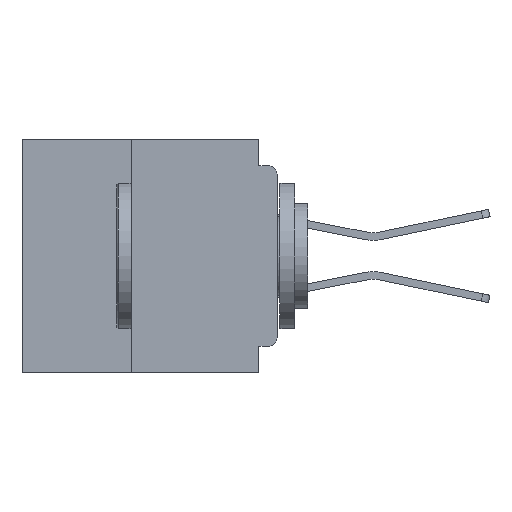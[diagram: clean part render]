
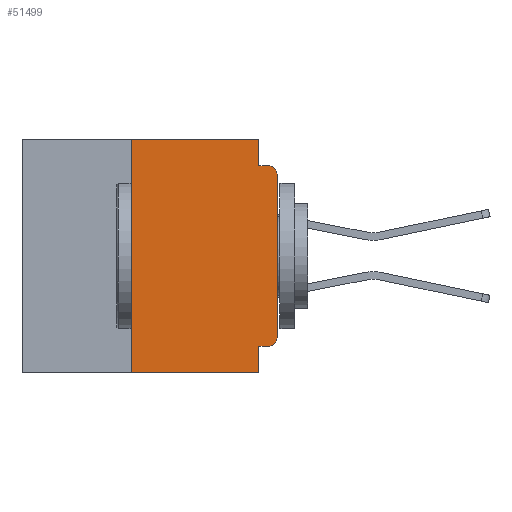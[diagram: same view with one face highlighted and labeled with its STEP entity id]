
A CAD part, left-side view. The second image highlights one B-rep face of the part: STEP entity #51499.
In plain terms, the highlighted planar face has unit normal (-1, 0, 0).
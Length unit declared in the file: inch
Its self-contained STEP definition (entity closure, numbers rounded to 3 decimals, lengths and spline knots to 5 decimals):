
#126 = CARTESIAN_POINT ( 'NONE',  ( 0., 0.031, 0. ) ) ;
#289 = LINE ( 'NONE', #2831, #24535 ) ;
#357 = EDGE_CURVE ( 'NONE', #18893, #23499, #23217, .T. ) ;
#676 = DIRECTION ( 'NONE',  ( -1., 0., 0. ) ) ;
#738 = CARTESIAN_POINT ( 'NONE',  ( 0., 0.25, -0.4 ) ) ;
#1469 = CARTESIAN_POINT ( 'NONE',  ( 0., 0.015, -0.06 ) ) ;
#1670 = EDGE_LOOP ( 'NONE', ( #58334, #9150, #5687, #19805, #4033, #35857, #39417, #44294, #11876, #18466 ) ) ;
#2831 = CARTESIAN_POINT ( 'NONE',  ( 0., 0.031, 0. ) ) ;
#4033 = ORIENTED_EDGE ( 'NONE', *, *, #4796, .F. ) ;
#4796 = EDGE_CURVE ( 'NONE', #25297, #15757, #52544, .T. ) ;
#5671 = CARTESIAN_POINT ( 'NONE',  ( 0., 0., 0. ) ) ;
#5687 = ORIENTED_EDGE ( 'NONE', *, *, #357, .F. ) ;
#6081 = DIRECTION ( 'NONE',  ( 0., 0., -1. ) ) ;
#9150 = ORIENTED_EDGE ( 'NONE', *, *, #38663, .T. ) ;
#9692 = DIRECTION ( 'NONE',  ( 1., 0., 0. ) ) ;
#10299 = DIRECTION ( 'NONE',  ( 0., 0., 1. ) ) ;
#10449 = DIRECTION ( 'NONE',  ( 0., -1., 0. ) ) ;
#11142 = DIRECTION ( 'NONE',  ( 0., -1., 0. ) ) ;
#11545 = CARTESIAN_POINT ( 'NONE',  ( 0., 0., -0.045 ) ) ;
#11761 = LINE ( 'NONE', #738, #20936 ) ;
#11876 = ORIENTED_EDGE ( 'NONE', *, *, #19337, .F. ) ;
#11877 = LINE ( 'NONE', #53021, #44969 ) ;
#12069 = VECTOR ( 'NONE', #54980, 39.37008 ) ;
#12243 = CARTESIAN_POINT ( 'NONE',  ( 0., 0.25, 0. ) ) ;
#12912 = VERTEX_POINT ( 'NONE', #33582 ) ;
#14119 = PLANE ( 'NONE',  #44494 ) ;
#14948 = CARTESIAN_POINT ( 'NONE',  ( 0., 0.25, -0.4 ) ) ;
#15237 = CARTESIAN_POINT ( 'NONE',  ( 0., 0., -0.34 ) ) ;
#15757 = VERTEX_POINT ( 'NONE', #126 ) ;
#16475 = AXIS2_PLACEMENT_3D ( 'NONE', #27942, #676, #32448 ) ;
#18466 = ORIENTED_EDGE ( 'NONE', *, *, #26228, .T. ) ;
#18893 = VERTEX_POINT ( 'NONE', #51088 ) ;
#19337 = EDGE_CURVE ( 'NONE', #45247, #51686, #29975, .T. ) ;
#19415 = VECTOR ( 'NONE', #10299, 39.37008 ) ;
#19533 = VERTEX_POINT ( 'NONE', #15237 ) ;
#19805 = ORIENTED_EDGE ( 'NONE', *, *, #40386, .F. ) ;
#20606 = CARTESIAN_POINT ( 'NONE',  ( 0., 0.031, -0.355 ) ) ;
#20936 = VECTOR ( 'NONE', #23467, 39.37008 ) ;
#21229 = CARTESIAN_POINT ( 'NONE',  ( 0., 0.015, -0.355 ) ) ;
#22928 = CARTESIAN_POINT ( 'NONE',  ( 0., 0., -0.06 ) ) ;
#23217 = LINE ( 'NONE', #11545, #35177 ) ;
#23467 = DIRECTION ( 'NONE',  ( 0., 0., 1. ) ) ;
#23499 = VERTEX_POINT ( 'NONE', #46255 ) ;
#24535 = VECTOR ( 'NONE', #34534, 39.37008 ) ;
#25297 = VERTEX_POINT ( 'NONE', #12243 ) ;
#26228 = EDGE_CURVE ( 'NONE', #45247, #19533, #51396, .T. ) ;
#27942 = CARTESIAN_POINT ( 'NONE',  ( 0., 0.015, -0.34 ) ) ;
#28572 = VECTOR ( 'NONE', #49833, 39.37008 ) ;
#29090 = VERTEX_POINT ( 'NONE', #22928 ) ;
#29975 = LINE ( 'NONE', #31791, #28572 ) ;
#30660 = DIRECTION ( 'NONE',  ( 0., 0., -1. ) ) ;
#31791 = CARTESIAN_POINT ( 'NONE',  ( 0., 0., -0.355 ) ) ;
#32448 = DIRECTION ( 'NONE',  ( 0., 0., -1. ) ) ;
#33213 = DIRECTION ( 'NONE',  ( -1., 0., 0. ) ) ;
#33582 = CARTESIAN_POINT ( 'NONE',  ( 0., 0.031, -0.4 ) ) ;
#34534 = DIRECTION ( 'NONE',  ( 0., 0., -1. ) ) ;
#35177 = VECTOR ( 'NONE', #11142, 39.37008 ) ;
#35857 = ORIENTED_EDGE ( 'NONE', *, *, #37922, .F. ) ;
#36954 = CARTESIAN_POINT ( 'NONE',  ( 0., 0.437, -0.4 ) ) ;
#37054 = EDGE_CURVE ( 'NONE', #51686, #12912, #11877, .T. ) ;
#37922 = EDGE_CURVE ( 'NONE', #39540, #25297, #11761, .T. ) ;
#38663 = EDGE_CURVE ( 'NONE', #29090, #23499, #39821, .T. ) ;
#39417 = ORIENTED_EDGE ( 'NONE', *, *, #45543, .T. ) ;
#39540 = VERTEX_POINT ( 'NONE', #14948 ) ;
#39821 = CIRCLE ( 'NONE', #47758, 0.015 ) ;
#40386 = EDGE_CURVE ( 'NONE', #15757, #18893, #289, .T. ) ;
#40548 = VECTOR ( 'NONE', #10449, 39.37008 ) ;
#41217 = DIRECTION ( 'NONE',  ( 0., 0., -1. ) ) ;
#44294 = ORIENTED_EDGE ( 'NONE', *, *, #37054, .F. ) ;
#44494 = AXIS2_PLACEMENT_3D ( 'NONE', #54577, #9692, #41217 ) ;
#44969 = VECTOR ( 'NONE', #30660, 39.37008 ) ;
#45247 = VERTEX_POINT ( 'NONE', #21229 ) ;
#45543 = EDGE_CURVE ( 'NONE', #39540, #12912, #47971, .T. ) ;
#46255 = CARTESIAN_POINT ( 'NONE',  ( 0., 0.015, -0.045 ) ) ;
#47758 = AXIS2_PLACEMENT_3D ( 'NONE', #1469, #33213, #6081 ) ;
#47813 = FACE_OUTER_BOUND ( 'NONE', #1670, .T. ) ;
#47971 = LINE ( 'NONE', #36954, #12069 ) ;
#49833 = DIRECTION ( 'NONE',  ( 0., 1., 0. ) ) ;
#50821 = CARTESIAN_POINT ( 'NONE',  ( 0., 0.437, 0. ) ) ;
#51088 = CARTESIAN_POINT ( 'NONE',  ( 0., 0.031, -0.045 ) ) ;
#51396 = CIRCLE ( 'NONE', #16475, 0.015 ) ;
#51499 = ADVANCED_FACE ( 'NONE', ( #47813 ), #14119, .F. ) ;
#51686 = VERTEX_POINT ( 'NONE', #20606 ) ;
#52544 = LINE ( 'NONE', #50821, #40548 ) ;
#53021 = CARTESIAN_POINT ( 'NONE',  ( 0., 0.031, -0.4 ) ) ;
#54431 = EDGE_CURVE ( 'NONE', #19533, #29090, #56655, .T. ) ;
#54577 = CARTESIAN_POINT ( 'NONE',  ( 0., 0.437, 0. ) ) ;
#54980 = DIRECTION ( 'NONE',  ( 0., -1., 0. ) ) ;
#56655 = LINE ( 'NONE', #5671, #19415 ) ;
#58334 = ORIENTED_EDGE ( 'NONE', *, *, #54431, .T. ) ;
